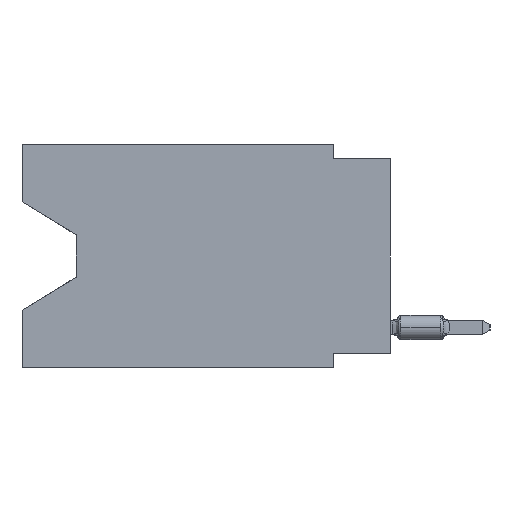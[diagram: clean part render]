
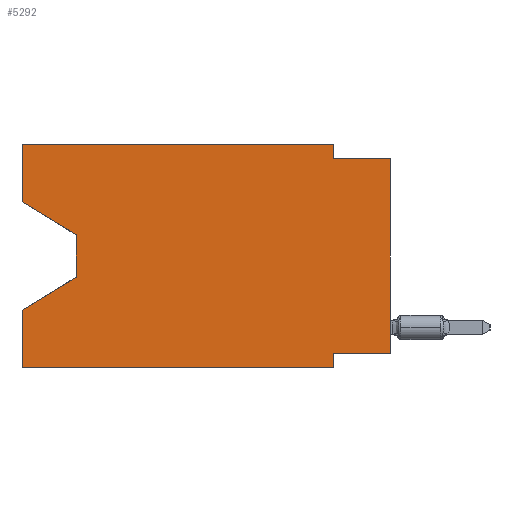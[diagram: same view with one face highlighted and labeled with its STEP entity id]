
A CAD part, left-side view. The second image highlights one B-rep face of the part: STEP entity #5292.
In plain terms, the highlighted planar face has unit normal (-1, 0, 0).
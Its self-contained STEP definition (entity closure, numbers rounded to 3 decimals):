
#854 = CARTESIAN_POINT ( 'NONE',  ( 0., 2.54, -9.271 ) ) ;
#2202 = EDGE_LOOP ( 'NONE', ( #7891, #36921, #13406, #23850, #21311, #31354, #26943, #37915, #17849, #20921, #21263, #2789 ) ) ;
#2789 = ORIENTED_EDGE ( 'NONE', *, *, #7624, .F. ) ;
#2952 = LINE ( 'NONE', #24698, #21122 ) ;
#3418 = CARTESIAN_POINT ( 'NONE',  ( 0., 13.97, -5.893 ) ) ;
#3420 = LINE ( 'NONE', #21926, #30921 ) ;
#4638 = VERTEX_POINT ( 'NONE', #18277 ) ;
#4779 = DIRECTION ( 'NONE',  ( 0., 0., -1. ) ) ;
#5031 = VERTEX_POINT ( 'NONE', #34281 ) ;
#5292 = ADVANCED_FACE ( 'NONE', ( #35681 ), #17775, .F. ) ;
#5329 = VERTEX_POINT ( 'NONE', #19115 ) ;
#5832 = VECTOR ( 'NONE', #16625, 1000. ) ;
#6995 = LINE ( 'NONE', #31983, #15341 ) ;
#7392 = EDGE_CURVE ( 'NONE', #13410, #7543, #37185, .T. ) ;
#7521 = CARTESIAN_POINT ( 'NONE',  ( 0., 16.383, -2.546 ) ) ;
#7543 = VERTEX_POINT ( 'NONE', #35142 ) ;
#7624 = EDGE_CURVE ( 'NONE', #8441, #4638, #26790, .T. ) ;
#7891 = ORIENTED_EDGE ( 'NONE', *, *, #38426, .T. ) ;
#8441 = VERTEX_POINT ( 'NONE', #7521 ) ;
#8980 = EDGE_CURVE ( 'NONE', #5329, #33003, #20275, .T. ) ;
#9170 = CARTESIAN_POINT ( 'NONE',  ( 0., 13.97, -4.013 ) ) ;
#9357 = VECTOR ( 'NONE', #36749, 1000. ) ;
#10551 = DIRECTION ( 'NONE',  ( 0., 0., -1. ) ) ;
#10571 = EDGE_CURVE ( 'NONE', #17682, #7543, #32713, .T. ) ;
#10851 = EDGE_CURVE ( 'NONE', #18880, #33003, #3420, .T. ) ;
#13406 = ORIENTED_EDGE ( 'NONE', *, *, #33076, .T. ) ;
#13410 = VERTEX_POINT ( 'NONE', #37671 ) ;
#13817 = CARTESIAN_POINT ( 'NONE',  ( 0., 0., -0.635 ) ) ;
#13860 = AXIS2_PLACEMENT_3D ( 'NONE', #20226, #32627, #4779 ) ;
#14220 = CARTESIAN_POINT ( 'NONE',  ( 0., 0., -9.271 ) ) ;
#14728 = VECTOR ( 'NONE', #17023, 1000. ) ;
#14796 = CARTESIAN_POINT ( 'NONE',  ( 0., 16.383, 0. ) ) ;
#15341 = VECTOR ( 'NONE', #31583, 1000. ) ;
#16625 = DIRECTION ( 'NONE',  ( 0., 0.855, -0.519 ) ) ;
#16839 = EDGE_CURVE ( 'NONE', #5329, #20740, #38809, .T. ) ;
#17023 = DIRECTION ( 'NONE',  ( 0., 0., 1. ) ) ;
#17254 = CARTESIAN_POINT ( 'NONE',  ( 0., 2.54, 0. ) ) ;
#17430 = CARTESIAN_POINT ( 'NONE',  ( 0., 16.383, -9.906 ) ) ;
#17682 = VERTEX_POINT ( 'NONE', #24008 ) ;
#17775 = PLANE ( 'NONE',  #13860 ) ;
#17849 = ORIENTED_EDGE ( 'NONE', *, *, #10571, .F. ) ;
#17853 = EDGE_CURVE ( 'NONE', #25656, #5031, #24353, .T. ) ;
#17873 = LINE ( 'NONE', #14220, #36089 ) ;
#18277 = CARTESIAN_POINT ( 'NONE',  ( 0., 16.383, 0. ) ) ;
#18880 = VERTEX_POINT ( 'NONE', #854 ) ;
#19115 = CARTESIAN_POINT ( 'NONE',  ( 0., 16.383, -9.906 ) ) ;
#19426 = EDGE_CURVE ( 'NONE', #4638, #36227, #2952, .T. ) ;
#20226 = CARTESIAN_POINT ( 'NONE',  ( 0., 16.383, 0. ) ) ;
#20275 = LINE ( 'NONE', #17430, #25439 ) ;
#20740 = VERTEX_POINT ( 'NONE', #27261 ) ;
#20921 = ORIENTED_EDGE ( 'NONE', *, *, #31556, .F. ) ;
#21122 = VECTOR ( 'NONE', #21653, 1000. ) ;
#21263 = ORIENTED_EDGE ( 'NONE', *, *, #19426, .F. ) ;
#21311 = ORIENTED_EDGE ( 'NONE', *, *, #8980, .T. ) ;
#21653 = DIRECTION ( 'NONE',  ( 0., -1., 0. ) ) ;
#21926 = CARTESIAN_POINT ( 'NONE',  ( 0., 2.54, -9.906 ) ) ;
#22453 = VECTOR ( 'NONE', #28231, 1000. ) ;
#22527 = LINE ( 'NONE', #3418, #5832 ) ;
#23137 = DIRECTION ( 'NONE',  ( 0., -1., 0. ) ) ;
#23850 = ORIENTED_EDGE ( 'NONE', *, *, #16839, .F. ) ;
#23992 = VECTOR ( 'NONE', #27211, 1000. ) ;
#24008 = CARTESIAN_POINT ( 'NONE',  ( 0., 2.54, -0.635 ) ) ;
#24353 = LINE ( 'NONE', #40011, #9357 ) ;
#24698 = CARTESIAN_POINT ( 'NONE',  ( 0., 16.383, 0. ) ) ;
#25439 = VECTOR ( 'NONE', #23137, 1000. ) ;
#25656 = VERTEX_POINT ( 'NONE', #9170 ) ;
#26790 = LINE ( 'NONE', #38985, #14728 ) ;
#26943 = ORIENTED_EDGE ( 'NONE', *, *, #39968, .F. ) ;
#27211 = DIRECTION ( 'NONE',  ( 0., 0., 1. ) ) ;
#27261 = CARTESIAN_POINT ( 'NONE',  ( 0., 16.383, -7.36 ) ) ;
#28043 = CARTESIAN_POINT ( 'NONE',  ( 0., 0., 0. ) ) ;
#28231 = DIRECTION ( 'NONE',  ( 0., 0., 1. ) ) ;
#28430 = DIRECTION ( 'NONE',  ( 0., 0., -1. ) ) ;
#28987 = VECTOR ( 'NONE', #30064, 1000. ) ;
#29453 = CARTESIAN_POINT ( 'NONE',  ( 0., 2.54, 0. ) ) ;
#30064 = DIRECTION ( 'NONE',  ( 0., -1., 0. ) ) ;
#30469 = CARTESIAN_POINT ( 'NONE',  ( 0., 2.54, -9.906 ) ) ;
#30921 = VECTOR ( 'NONE', #28430, 1000. ) ;
#31354 = ORIENTED_EDGE ( 'NONE', *, *, #10851, .F. ) ;
#31556 = EDGE_CURVE ( 'NONE', #36227, #17682, #38419, .T. ) ;
#31583 = DIRECTION ( 'NONE',  ( 0., -0.855, -0.519 ) ) ;
#31983 = CARTESIAN_POINT ( 'NONE',  ( 0., 16.383, -2.546 ) ) ;
#32627 = DIRECTION ( 'NONE',  ( 1., 0., 0. ) ) ;
#32713 = LINE ( 'NONE', #13817, #28987 ) ;
#33003 = VERTEX_POINT ( 'NONE', #30469 ) ;
#33076 = EDGE_CURVE ( 'NONE', #5031, #20740, #22527, .T. ) ;
#34281 = CARTESIAN_POINT ( 'NONE',  ( 0., 13.97, -5.893 ) ) ;
#35142 = CARTESIAN_POINT ( 'NONE',  ( 0., 0., -0.635 ) ) ;
#35681 = FACE_OUTER_BOUND ( 'NONE', #2202, .T. ) ;
#36089 = VECTOR ( 'NONE', #39028, 1000. ) ;
#36227 = VERTEX_POINT ( 'NONE', #17254 ) ;
#36749 = DIRECTION ( 'NONE',  ( 0., 0., -1. ) ) ;
#36921 = ORIENTED_EDGE ( 'NONE', *, *, #17853, .T. ) ;
#37185 = LINE ( 'NONE', #28043, #22453 ) ;
#37671 = CARTESIAN_POINT ( 'NONE',  ( 0., 0., -9.271 ) ) ;
#37915 = ORIENTED_EDGE ( 'NONE', *, *, #7392, .T. ) ;
#38419 = LINE ( 'NONE', #29453, #38847 ) ;
#38426 = EDGE_CURVE ( 'NONE', #8441, #25656, #6995, .T. ) ;
#38809 = LINE ( 'NONE', #14796, #23992 ) ;
#38847 = VECTOR ( 'NONE', #10551, 1000. ) ;
#38985 = CARTESIAN_POINT ( 'NONE',  ( 0., 16.383, 0. ) ) ;
#39028 = DIRECTION ( 'NONE',  ( 0., 1., 0. ) ) ;
#39968 = EDGE_CURVE ( 'NONE', #13410, #18880, #17873, .T. ) ;
#40011 = CARTESIAN_POINT ( 'NONE',  ( 0., 13.97, -4.013 ) ) ;
